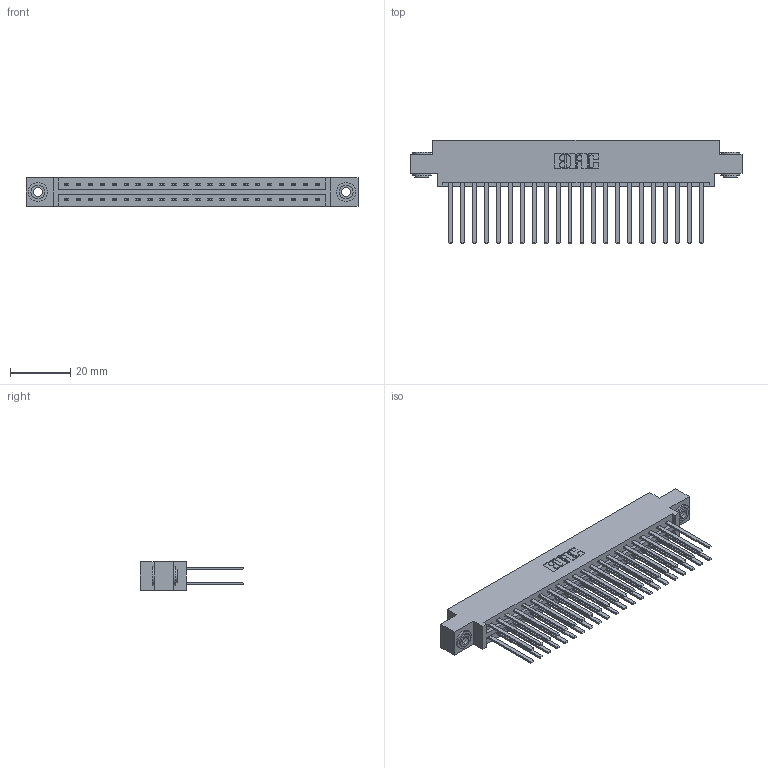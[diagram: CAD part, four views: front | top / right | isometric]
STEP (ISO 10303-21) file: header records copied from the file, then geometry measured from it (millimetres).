
FILE_DESCRIPTION (( 'STEP AP203' ), '1' );
FILE_NAME ('387-044-544-803.STEP', '2018-09-20T02:32:24', ( '' ), ( '' ), 'SwSTEP 2.0', 'SolidWorks 2016', '' );
FILE_SCHEMA (( 'CONFIG_CONTROL_DESIGN' ));
Length unit declared in the file: inch
Products named in the file (4): 337 Part_0.170 Offset - 0.156 Dia-TH; 345-292-001_345-293-144; 345-250-002_345-250-002-102; 387-044-544-803
Assembly tree (47 placements, depth 2):
  387-044-544-803
    337 Part_0.170 Offset - 0.156 Dia-TH
    345-292-001_345-293-144  x44
    345-250-002_345-250-002-102  x2
Bounding box: 110.19 x 34.3 x 9.4 mm (x, y, z)
Volume: 11864.7 mm3; surface area: 15565.9 mm2
Topology: 47 solids, 47 shells, 2268 faces, 6691 edges, 4398 vertices
Faces by surface type: plane 1580, cylinder 680, cone 8
Entity records: 20242 total; most frequent: CARTESIAN_POINT 3401, ORIENTED_EDGE 3330, DIRECTION 2959, EDGE_CURVE 1665, VECTOR 1517, LINE 1517, VERTEX_POINT 1106, AXIS2_PLACEMENT_3D 721
